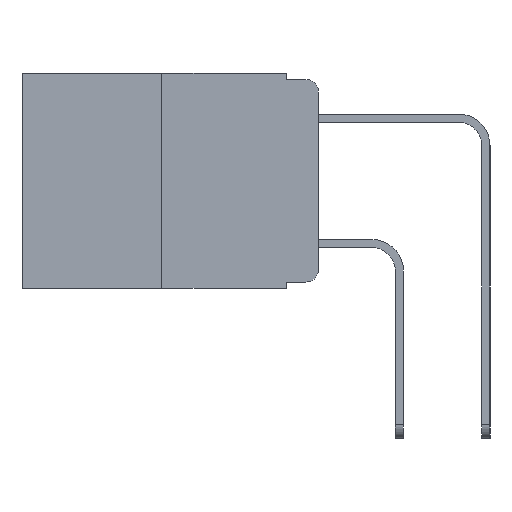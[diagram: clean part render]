
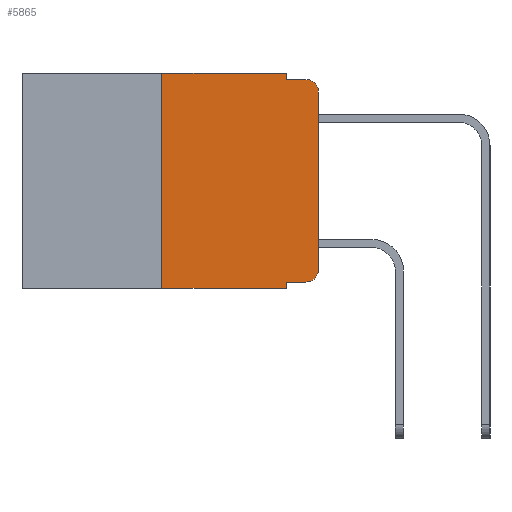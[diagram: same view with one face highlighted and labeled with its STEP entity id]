
A CAD part, left-side view. The second image highlights one B-rep face of the part: STEP entity #5865.
In plain terms, the highlighted planar face has unit normal (-1, 0, 0).
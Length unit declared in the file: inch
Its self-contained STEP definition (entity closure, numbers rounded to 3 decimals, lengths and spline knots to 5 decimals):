
#68 = EDGE_CURVE ( 'NONE', #176, #9299, #13706, .T. ) ;
#120 = CARTESIAN_POINT ( 'NONE',  ( 0., 0.02, -0.01 ) ) ;
#176 = VERTEX_POINT ( 'NONE', #3482 ) ;
#184 = CIRCLE ( 'NONE', #15447, 0.02 ) ;
#201 = CIRCLE ( 'NONE', #7254, 0.02 ) ;
#235 = CARTESIAN_POINT ( 'NONE',  ( 0., 0.051, -0.343 ) ) ;
#238 = DIRECTION ( 'NONE',  ( -1., 0., 0. ) ) ;
#325 = CARTESIAN_POINT ( 'NONE',  ( 0., 0.051, -0.333 ) ) ;
#900 = DIRECTION ( 'NONE',  ( 0., 0., 1. ) ) ;
#1050 = AXIS2_PLACEMENT_3D ( 'NONE', #7918, #10406, #2972 ) ;
#1179 = LINE ( 'NONE', #1428, #7039 ) ;
#1352 = LINE ( 'NONE', #10910, #1757 ) ;
#1428 = CARTESIAN_POINT ( 'NONE',  ( 0., 0.051, -0.01 ) ) ;
#1757 = VECTOR ( 'NONE', #900, 39.37008 ) ;
#2144 = CARTESIAN_POINT ( 'NONE',  ( 0., 0.25, -0.343 ) ) ;
#2211 = CARTESIAN_POINT ( 'NONE',  ( 0., 0.473, 0. ) ) ;
#2430 = ORIENTED_EDGE ( 'NONE', *, *, #14547, .F. ) ;
#2494 = LINE ( 'NONE', #2211, #15532 ) ;
#2587 = ORIENTED_EDGE ( 'NONE', *, *, #5521, .T. ) ;
#2972 = DIRECTION ( 'NONE',  ( 0., 0., -1. ) ) ;
#3188 = VECTOR ( 'NONE', #3771, 39.37008 ) ;
#3324 = VECTOR ( 'NONE', #3697, 39.37008 ) ;
#3445 = EDGE_CURVE ( 'NONE', #5507, #3844, #13991, .T. ) ;
#3482 = CARTESIAN_POINT ( 'NONE',  ( 0., 0.051, -0.333 ) ) ;
#3505 = DIRECTION ( 'NONE',  ( 0., -1., 0. ) ) ;
#3697 = DIRECTION ( 'NONE',  ( 0., 0., -1. ) ) ;
#3731 = DIRECTION ( 'NONE',  ( 0., 0., -1. ) ) ;
#3771 = DIRECTION ( 'NONE',  ( 0., -1., 0. ) ) ;
#3844 = VERTEX_POINT ( 'NONE', #13676 ) ;
#4148 = ORIENTED_EDGE ( 'NONE', *, *, #10532, .T. ) ;
#4180 = ORIENTED_EDGE ( 'NONE', *, *, #15237, .T. ) ;
#4287 = ORIENTED_EDGE ( 'NONE', *, *, #68, .T. ) ;
#4329 = CARTESIAN_POINT ( 'NONE',  ( 0., 0.02, -0.313 ) ) ;
#4502 = ORIENTED_EDGE ( 'NONE', *, *, #13946, .F. ) ;
#4731 = ORIENTED_EDGE ( 'NONE', *, *, #9027, .T. ) ;
#4803 = ORIENTED_EDGE ( 'NONE', *, *, #3445, .F. ) ;
#5129 = CARTESIAN_POINT ( 'NONE',  ( 0., 0., -0.03 ) ) ;
#5507 = VERTEX_POINT ( 'NONE', #2144 ) ;
#5521 = EDGE_CURVE ( 'NONE', #7474, #15006, #1352, .T. ) ;
#5526 = DIRECTION ( 'NONE',  ( 0., 0., -1. ) ) ;
#5784 = ORIENTED_EDGE ( 'NONE', *, *, #15437, .F. ) ;
#5853 = CARTESIAN_POINT ( 'NONE',  ( 0., 0., -0.313 ) ) ;
#5865 = ADVANCED_FACE ( 'NONE', ( #11662 ), #9190, .F. ) ;
#6165 = CARTESIAN_POINT ( 'NONE',  ( 0., 0.051, 0. ) ) ;
#6776 = CARTESIAN_POINT ( 'NONE',  ( 0., 0.051, -0.01 ) ) ;
#7039 = VECTOR ( 'NONE', #8937, 39.37008 ) ;
#7254 = AXIS2_PLACEMENT_3D ( 'NONE', #7699, #238, #8974 ) ;
#7474 = VERTEX_POINT ( 'NONE', #5853 ) ;
#7699 = CARTESIAN_POINT ( 'NONE',  ( 0., 0.02, -0.03 ) ) ;
#7879 = DIRECTION ( 'NONE',  ( 0., 0., 1. ) ) ;
#7918 = CARTESIAN_POINT ( 'NONE',  ( 0., 0.473, 0. ) ) ;
#8084 = EDGE_LOOP ( 'NONE', ( #2587, #4148, #2430, #5784, #8827, #4803, #4731, #4502, #4287, #4180 ) ) ;
#8092 = VECTOR ( 'NONE', #3731, 39.37008 ) ;
#8496 = LINE ( 'NONE', #15882, #8092 ) ;
#8710 = CARTESIAN_POINT ( 'NONE',  ( 0., 0.473, -0.343 ) ) ;
#8827 = ORIENTED_EDGE ( 'NONE', *, *, #11986, .F. ) ;
#8937 = DIRECTION ( 'NONE',  ( 0., -1., 0. ) ) ;
#8974 = DIRECTION ( 'NONE',  ( 0., 0., -1. ) ) ;
#9027 = EDGE_CURVE ( 'NONE', #5507, #15554, #10188, .T. ) ;
#9068 = CARTESIAN_POINT ( 'NONE',  ( 0., 0.02, -0.333 ) ) ;
#9190 = PLANE ( 'NONE',  #1050 ) ;
#9299 = VERTEX_POINT ( 'NONE', #9068 ) ;
#9690 = DIRECTION ( 'NONE',  ( 0., -1., 0. ) ) ;
#10050 = VERTEX_POINT ( 'NONE', #6776 ) ;
#10188 = LINE ( 'NONE', #8710, #3188 ) ;
#10406 = DIRECTION ( 'NONE',  ( 1., 0., 0. ) ) ;
#10491 = VERTEX_POINT ( 'NONE', #120 ) ;
#10509 = VECTOR ( 'NONE', #3505, 39.37008 ) ;
#10532 = EDGE_CURVE ( 'NONE', #15006, #10491, #201, .T. ) ;
#10910 = CARTESIAN_POINT ( 'NONE',  ( 0., 0., 0. ) ) ;
#11537 = CARTESIAN_POINT ( 'NONE',  ( 0., 0.25, 0. ) ) ;
#11662 = FACE_OUTER_BOUND ( 'NONE', #8084, .T. ) ;
#11986 = EDGE_CURVE ( 'NONE', #3844, #15201, #2494, .T. ) ;
#12905 = DIRECTION ( 'NONE',  ( -1., 0., 0. ) ) ;
#13154 = LINE ( 'NONE', #6165, #3324 ) ;
#13676 = CARTESIAN_POINT ( 'NONE',  ( 0., 0.25, 0. ) ) ;
#13706 = LINE ( 'NONE', #325, #10509 ) ;
#13946 = EDGE_CURVE ( 'NONE', #176, #15554, #8496, .T. ) ;
#13991 = LINE ( 'NONE', #11537, #14722 ) ;
#14547 = EDGE_CURVE ( 'NONE', #10050, #10491, #1179, .T. ) ;
#14722 = VECTOR ( 'NONE', #7879, 39.37008 ) ;
#15006 = VERTEX_POINT ( 'NONE', #5129 ) ;
#15201 = VERTEX_POINT ( 'NONE', #15202 ) ;
#15202 = CARTESIAN_POINT ( 'NONE',  ( 0., 0.051, 0. ) ) ;
#15237 = EDGE_CURVE ( 'NONE', #9299, #7474, #184, .T. ) ;
#15437 = EDGE_CURVE ( 'NONE', #15201, #10050, #13154, .T. ) ;
#15447 = AXIS2_PLACEMENT_3D ( 'NONE', #4329, #12905, #5526 ) ;
#15532 = VECTOR ( 'NONE', #9690, 39.37008 ) ;
#15554 = VERTEX_POINT ( 'NONE', #235 ) ;
#15882 = CARTESIAN_POINT ( 'NONE',  ( 0., 0.051, 0. ) ) ;
